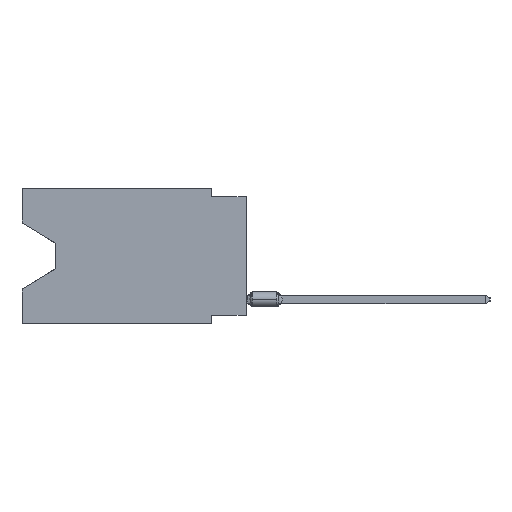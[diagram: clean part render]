
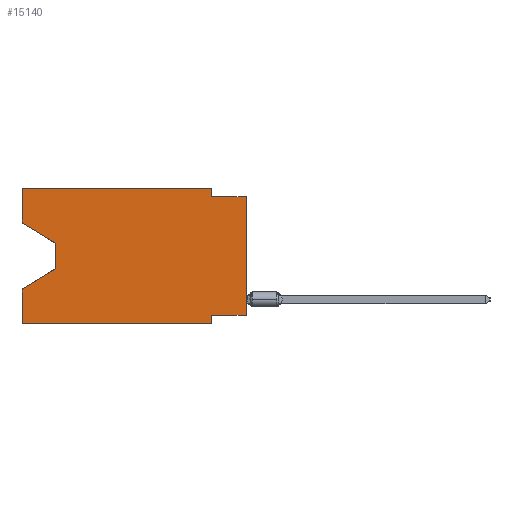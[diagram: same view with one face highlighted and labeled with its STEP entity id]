
A CAD part, left-side view. The second image highlights one B-rep face of the part: STEP entity #15140.
In plain terms, the highlighted planar face has unit normal (-1, 0, 0).
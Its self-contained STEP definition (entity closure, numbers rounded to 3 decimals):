
#615 = VERTEX_POINT ( 'NONE', #24306 ) ;
#625 = VERTEX_POINT ( 'NONE', #37115 ) ;
#729 = FACE_OUTER_BOUND ( 'NONE', #38615, .T. ) ;
#869 = CARTESIAN_POINT ( 'NONE',  ( 0., 16.383, -2.546 ) ) ;
#1125 = VECTOR ( 'NONE', #6634, 1000. ) ;
#1566 = VERTEX_POINT ( 'NONE', #9840 ) ;
#3293 = CARTESIAN_POINT ( 'NONE',  ( 0., 16.383, 0. ) ) ;
#3533 = DIRECTION ( 'NONE',  ( 0., 0., 1. ) ) ;
#4559 = LINE ( 'NONE', #10453, #24744 ) ;
#5142 = EDGE_CURVE ( 'NONE', #40570, #8754, #4559, .T. ) ;
#5556 = LINE ( 'NONE', #30988, #17745 ) ;
#5619 = DIRECTION ( 'NONE',  ( 0., -1., 0. ) ) ;
#6423 = LINE ( 'NONE', #38584, #1125 ) ;
#6469 = LINE ( 'NONE', #10026, #21201 ) ;
#6560 = ORIENTED_EDGE ( 'NONE', *, *, #5142, .T. ) ;
#6634 = DIRECTION ( 'NONE',  ( 0., -1., 0. ) ) ;
#6707 = CARTESIAN_POINT ( 'NONE',  ( 0., 16.383, -7.36 ) ) ;
#6879 = EDGE_CURVE ( 'NONE', #625, #16873, #9373, .T. ) ;
#6963 = DIRECTION ( 'NONE',  ( 0., 0., 1. ) ) ;
#7283 = LINE ( 'NONE', #13203, #34494 ) ;
#7457 = CARTESIAN_POINT ( 'NONE',  ( 0., 16.383, 0. ) ) ;
#7565 = VECTOR ( 'NONE', #30144, 1000. ) ;
#7592 = ORIENTED_EDGE ( 'NONE', *, *, #34150, .T. ) ;
#8123 = ORIENTED_EDGE ( 'NONE', *, *, #21061, .F. ) ;
#8300 = ORIENTED_EDGE ( 'NONE', *, *, #39020, .F. ) ;
#8439 = VECTOR ( 'NONE', #40040, 1000. ) ;
#8754 = VERTEX_POINT ( 'NONE', #6707 ) ;
#9303 = EDGE_CURVE ( 'NONE', #16873, #27778, #23646, .T. ) ;
#9373 = LINE ( 'NONE', #16312, #26176 ) ;
#9840 = CARTESIAN_POINT ( 'NONE',  ( 0., 16.383, -9.906 ) ) ;
#9931 = CARTESIAN_POINT ( 'NONE',  ( 0., 2.54, -0.635 ) ) ;
#10026 = CARTESIAN_POINT ( 'NONE',  ( 0., 0., 0. ) ) ;
#10204 = AXIS2_PLACEMENT_3D ( 'NONE', #7457, #13557, #32881 ) ;
#10453 = CARTESIAN_POINT ( 'NONE',  ( 0., 13.97, -5.893 ) ) ;
#10971 = CARTESIAN_POINT ( 'NONE',  ( 0., 2.54, 0. ) ) ;
#11258 = EDGE_CURVE ( 'NONE', #1566, #8754, #22942, .T. ) ;
#12149 = LINE ( 'NONE', #34408, #37393 ) ;
#12555 = VERTEX_POINT ( 'NONE', #20765 ) ;
#12974 = DIRECTION ( 'NONE',  ( 0., -1., 0. ) ) ;
#13203 = CARTESIAN_POINT ( 'NONE',  ( 0., 13.97, -4.013 ) ) ;
#13557 = DIRECTION ( 'NONE',  ( 1., 0., 0. ) ) ;
#14693 = CARTESIAN_POINT ( 'NONE',  ( 0., 2.54, -9.906 ) ) ;
#15140 = ADVANCED_FACE ( 'NONE', ( #729 ), #36455, .F. ) ;
#15620 = EDGE_CURVE ( 'NONE', #615, #32141, #39975, .T. ) ;
#16312 = CARTESIAN_POINT ( 'NONE',  ( 0., 0., -9.271 ) ) ;
#16873 = VERTEX_POINT ( 'NONE', #40468 ) ;
#17556 = EDGE_CURVE ( 'NONE', #34754, #12555, #5556, .T. ) ;
#17745 = VECTOR ( 'NONE', #25328, 1000. ) ;
#19070 = CARTESIAN_POINT ( 'NONE',  ( 0., 0., -0.635 ) ) ;
#20083 = ORIENTED_EDGE ( 'NONE', *, *, #15620, .F. ) ;
#20090 = LINE ( 'NONE', #30571, #8439 ) ;
#20765 = CARTESIAN_POINT ( 'NONE',  ( 0., 13.97, -4.013 ) ) ;
#21061 = EDGE_CURVE ( 'NONE', #32141, #29895, #23387, .T. ) ;
#21201 = VECTOR ( 'NONE', #3533, 1000. ) ;
#21232 = VERTEX_POINT ( 'NONE', #3293 ) ;
#22200 = DIRECTION ( 'NONE',  ( 0., 1., 0. ) ) ;
#22942 = LINE ( 'NONE', #38503, #24078 ) ;
#23387 = LINE ( 'NONE', #19070, #26293 ) ;
#23646 = LINE ( 'NONE', #28199, #7565 ) ;
#23687 = DIRECTION ( 'NONE',  ( 0., 0.855, -0.519 ) ) ;
#23702 = EDGE_CURVE ( 'NONE', #12555, #40570, #7283, .T. ) ;
#23795 = DIRECTION ( 'NONE',  ( 0., 0., -1. ) ) ;
#24078 = VECTOR ( 'NONE', #6963, 1000. ) ;
#24306 = CARTESIAN_POINT ( 'NONE',  ( 0., 2.54, 0. ) ) ;
#24744 = VECTOR ( 'NONE', #23687, 1000. ) ;
#25054 = ORIENTED_EDGE ( 'NONE', *, *, #28442, .T. ) ;
#25317 = ORIENTED_EDGE ( 'NONE', *, *, #6879, .F. ) ;
#25328 = DIRECTION ( 'NONE',  ( 0., -0.855, -0.519 ) ) ;
#26018 = DIRECTION ( 'NONE',  ( 0., 0., -1. ) ) ;
#26066 = CARTESIAN_POINT ( 'NONE',  ( 0., 0., -0.635 ) ) ;
#26176 = VECTOR ( 'NONE', #22200, 1000. ) ;
#26293 = VECTOR ( 'NONE', #12974, 1000. ) ;
#27778 = VERTEX_POINT ( 'NONE', #14693 ) ;
#28199 = CARTESIAN_POINT ( 'NONE',  ( 0., 2.54, -9.906 ) ) ;
#28242 = ORIENTED_EDGE ( 'NONE', *, *, #17556, .T. ) ;
#28442 = EDGE_CURVE ( 'NONE', #1566, #27778, #6423, .T. ) ;
#29882 = ORIENTED_EDGE ( 'NONE', *, *, #37432, .F. ) ;
#29895 = VERTEX_POINT ( 'NONE', #26066 ) ;
#30144 = DIRECTION ( 'NONE',  ( 0., 0., -1. ) ) ;
#30571 = CARTESIAN_POINT ( 'NONE',  ( 0., 16.383, 0. ) ) ;
#30988 = CARTESIAN_POINT ( 'NONE',  ( 0., 16.383, -2.546 ) ) ;
#31748 = ORIENTED_EDGE ( 'NONE', *, *, #11258, .F. ) ;
#32141 = VERTEX_POINT ( 'NONE', #9931 ) ;
#32881 = DIRECTION ( 'NONE',  ( 0., 0., -1. ) ) ;
#34150 = EDGE_CURVE ( 'NONE', #625, #29895, #6469, .T. ) ;
#34408 = CARTESIAN_POINT ( 'NONE',  ( 0., 16.383, 0. ) ) ;
#34494 = VECTOR ( 'NONE', #26018, 1000. ) ;
#34754 = VERTEX_POINT ( 'NONE', #869 ) ;
#35413 = ORIENTED_EDGE ( 'NONE', *, *, #23702, .T. ) ;
#35741 = VECTOR ( 'NONE', #23795, 1000. ) ;
#36455 = PLANE ( 'NONE',  #10204 ) ;
#37115 = CARTESIAN_POINT ( 'NONE',  ( 0., 0., -9.271 ) ) ;
#37202 = ORIENTED_EDGE ( 'NONE', *, *, #9303, .F. ) ;
#37393 = VECTOR ( 'NONE', #5619, 1000. ) ;
#37432 = EDGE_CURVE ( 'NONE', #34754, #21232, #20090, .T. ) ;
#37913 = CARTESIAN_POINT ( 'NONE',  ( 0., 13.97, -5.893 ) ) ;
#38503 = CARTESIAN_POINT ( 'NONE',  ( 0., 16.383, 0. ) ) ;
#38584 = CARTESIAN_POINT ( 'NONE',  ( 0., 16.383, -9.906 ) ) ;
#38615 = EDGE_LOOP ( 'NONE', ( #28242, #35413, #6560, #31748, #25054, #37202, #25317, #7592, #8123, #20083, #8300, #29882 ) ) ;
#39020 = EDGE_CURVE ( 'NONE', #21232, #615, #12149, .T. ) ;
#39975 = LINE ( 'NONE', #10971, #35741 ) ;
#40040 = DIRECTION ( 'NONE',  ( 0., 0., 1. ) ) ;
#40468 = CARTESIAN_POINT ( 'NONE',  ( 0., 2.54, -9.271 ) ) ;
#40570 = VERTEX_POINT ( 'NONE', #37913 ) ;
